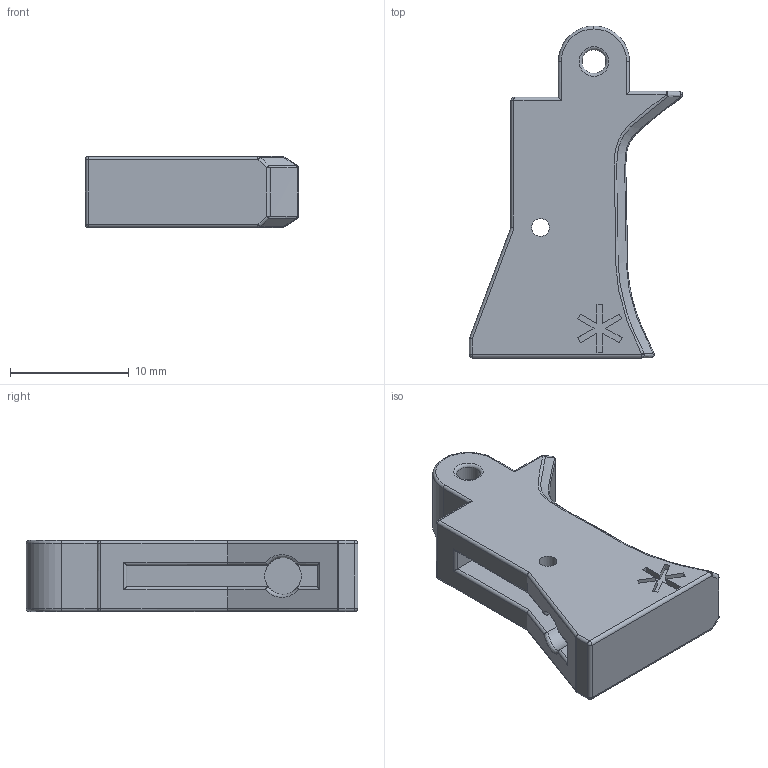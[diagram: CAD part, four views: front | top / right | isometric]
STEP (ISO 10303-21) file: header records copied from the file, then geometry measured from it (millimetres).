
FILE_DESCRIPTION(('HOOPS Exchange Step'),'2;1');
FILE_NAME('temp_export','2020-12-20T21:01:32+19:00',('mobile'),('Shapr3D Limited'),'HOOPS Exchange 2020.2','Shapr3D','Authorized');
FILE_SCHEMA( ('AP203_CONFIGURATION_CONTROLLED_3D_DESIGN_OF_MECHANICAL_PARTS_AND_ASSEMBLIES_MIM_LF') );
Length unit declared in the file: millimetre
Products named in the file (5): 0; CC46C01C-16ED-48DF-A70E-68239DD8D809.tmp
Assembly tree (4 placements, depth 2):
  CC46C01C-16ED-48DF-A70E-68239DD8D809.tmp
    0
    0
    0
    0
Bounding box: 17.98 x 28 x 6 mm (x, y, z)
Volume: 1451.9 mm3; surface area: 1368.2 mm2
Topology: 1 solids, 1 shells, 133 faces, 347 edges, 206 vertices
Faces by surface type: plane 57, cylinder 35, sphere 18, bspline 15, torus 8
Full cylindrical faces by diameter (mm): 1.5 x2, 2 x1, 3.1 x1
Entity records: 7086 total; most frequent: CARTESIAN_POINT 3793, DIRECTION 677, ORIENTED_EDGE 670, EDGE_CURVE 335, AXIS2_PLACEMENT_3D 243, VERTEX_POINT 206, VECTOR 191, LINE 191
